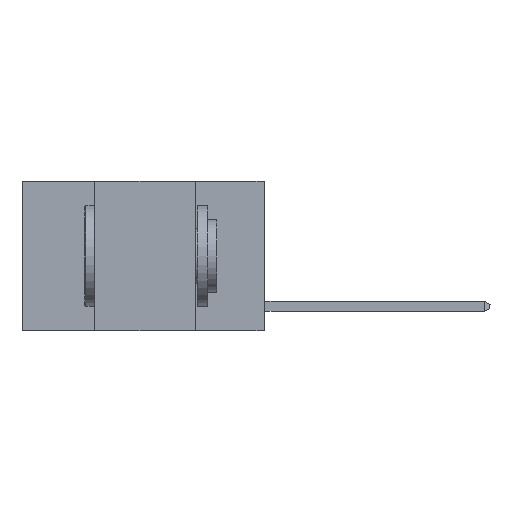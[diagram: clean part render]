
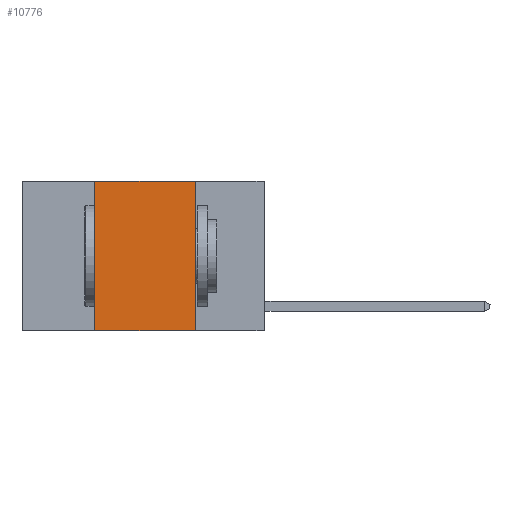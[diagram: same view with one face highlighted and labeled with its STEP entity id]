
A CAD part, left-side view. The second image highlights one B-rep face of the part: STEP entity #10776.
In plain terms, the highlighted planar face has unit normal (-1, 0, 0).
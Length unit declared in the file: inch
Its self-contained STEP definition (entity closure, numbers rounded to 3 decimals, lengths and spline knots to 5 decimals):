
#12 = CARTESIAN_POINT ( 'NONE',  ( 0., 0.6, -0.37 ) ) ;
#119 = ORIENTED_EDGE ( 'NONE', *, *, #653, .F. ) ;
#273 = CARTESIAN_POINT ( 'NONE',  ( 0., 0.42, 0. ) ) ;
#653 = EDGE_CURVE ( 'NONE', #10722, #7356, #2397, .T. ) ;
#1151 = CARTESIAN_POINT ( 'NONE',  ( 0., 0.6, 0. ) ) ;
#1320 = DIRECTION ( 'NONE',  ( 1., 0., 0. ) ) ;
#2071 = DIRECTION ( 'NONE',  ( 0., 0., 1. ) ) ;
#2205 = DIRECTION ( 'NONE',  ( 0., -1., 0. ) ) ;
#2242 = DIRECTION ( 'NONE',  ( 0., -1., 0. ) ) ;
#2397 = LINE ( 'NONE', #273, #9989 ) ;
#2574 = CARTESIAN_POINT ( 'NONE',  ( 0., 0.17, -0.37 ) ) ;
#3230 = CARTESIAN_POINT ( 'NONE',  ( 0., 0.6, 0. ) ) ;
#3648 = LINE ( 'NONE', #12, #4735 ) ;
#3991 = ORIENTED_EDGE ( 'NONE', *, *, #10473, .F. ) ;
#4116 = CARTESIAN_POINT ( 'NONE',  ( 0., 0.42, -0.37 ) ) ;
#4666 = EDGE_CURVE ( 'NONE', #6303, #10507, #7517, .T. ) ;
#4735 = VECTOR ( 'NONE', #2242, 39.37008 ) ;
#4950 = CARTESIAN_POINT ( 'NONE',  ( 0., 0.17, 0. ) ) ;
#5035 = ORIENTED_EDGE ( 'NONE', *, *, #4666, .F. ) ;
#5976 = CARTESIAN_POINT ( 'NONE',  ( 0., 0.17, 0. ) ) ;
#6140 = PLANE ( 'NONE',  #7137 ) ;
#6303 = VERTEX_POINT ( 'NONE', #5976 ) ;
#6820 = EDGE_LOOP ( 'NONE', ( #5035, #3991, #119, #12715 ) ) ;
#7001 = DIRECTION ( 'NONE',  ( 0., 0., -1. ) ) ;
#7137 = AXIS2_PLACEMENT_3D ( 'NONE', #1151, #1320, #12102 ) ;
#7259 = VECTOR ( 'NONE', #2205, 39.37008 ) ;
#7356 = VERTEX_POINT ( 'NONE', #8530 ) ;
#7517 = LINE ( 'NONE', #4950, #9972 ) ;
#8486 = LINE ( 'NONE', #3230, #7259 ) ;
#8530 = CARTESIAN_POINT ( 'NONE',  ( 0., 0.42, 0. ) ) ;
#9885 = EDGE_CURVE ( 'NONE', #10722, #10507, #3648, .T. ) ;
#9972 = VECTOR ( 'NONE', #7001, 39.37008 ) ;
#9989 = VECTOR ( 'NONE', #2071, 39.37008 ) ;
#10473 = EDGE_CURVE ( 'NONE', #7356, #6303, #8486, .T. ) ;
#10507 = VERTEX_POINT ( 'NONE', #2574 ) ;
#10722 = VERTEX_POINT ( 'NONE', #4116 ) ;
#10768 = FACE_OUTER_BOUND ( 'NONE', #6820, .T. ) ;
#10776 = ADVANCED_FACE ( 'NONE', ( #10768 ), #6140, .F. ) ;
#12102 = DIRECTION ( 'NONE',  ( 0., 0., -1. ) ) ;
#12715 = ORIENTED_EDGE ( 'NONE', *, *, #9885, .T. ) ;
